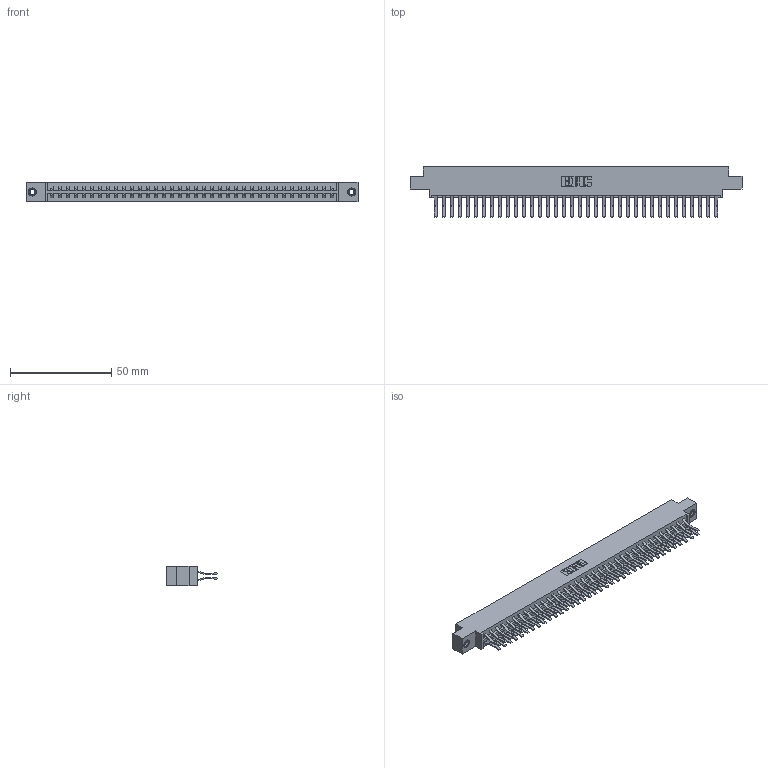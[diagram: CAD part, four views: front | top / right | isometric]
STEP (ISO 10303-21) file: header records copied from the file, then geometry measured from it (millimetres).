
FILE_DESCRIPTION (( 'STEP AP203' ), '1' );
FILE_NAME ('833-072-560-807.STEP', '2020-06-05T15:19:44', ( '' ), ( '' ), 'SwSTEP 2.0', 'SolidWorks 2020', '' );
FILE_SCHEMA (( 'CONFIG_CONTROL_DESIGN' ));
Length unit declared in the file: inch
Products named in the file (4): 833-072-560-807; 345-292-001_560 Tail; 833 Part_Offset - .156 Dia - TI; 345-250-001_345-250-005-103
Assembly tree (75 placements, depth 2):
  833-072-560-807
    833 Part_Offset - .156 Dia - TI
    345-292-001_560 Tail  x72
    345-250-001_345-250-005-103  x2
Bounding box: 164.19 x 24.78 x 9.4 mm (x, y, z)
Volume: 16936.9 mm3; surface area: 21560.4 mm2
Topology: 75 solids, 75 shells, 4066 faces, 12051 edges, 7930 vertices
Faces by surface type: plane 2698, cylinder 1352, cone 12, torus 4
Entity records: 25342 total; most frequent: CARTESIAN_POINT 4193, ORIENTED_EDGE 4122, DIRECTION 3627, EDGE_CURVE 2061, LINE 1909, VECTOR 1909, VERTEX_POINT 1368, AXIS2_PLACEMENT_3D 859
